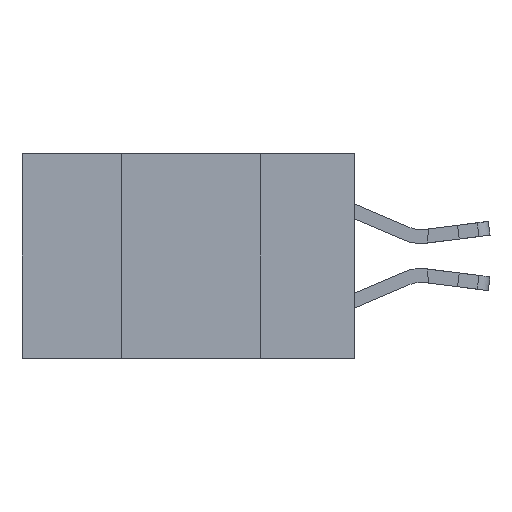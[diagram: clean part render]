
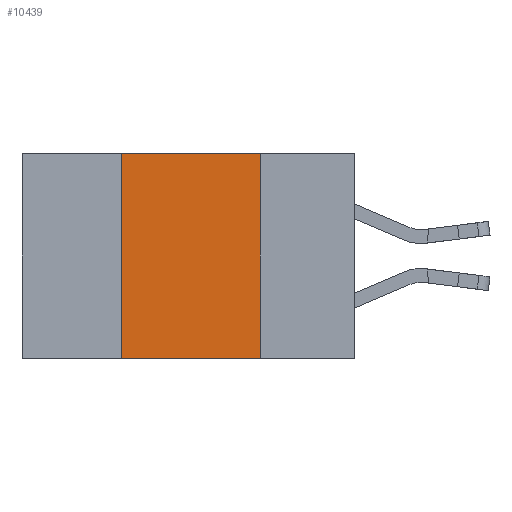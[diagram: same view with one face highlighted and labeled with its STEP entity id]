
A CAD part, left-side view. The second image highlights one B-rep face of the part: STEP entity #10439.
In plain terms, the highlighted planar face has unit normal (-1, 0, 0).
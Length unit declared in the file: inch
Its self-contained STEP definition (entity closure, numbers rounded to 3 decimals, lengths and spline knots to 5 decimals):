
#597 = CARTESIAN_POINT ( 'NONE',  ( 0., 0.42, -0.37 ) ) ;
#1867 = VERTEX_POINT ( 'NONE', #4042 ) ;
#1961 = CARTESIAN_POINT ( 'NONE',  ( 0., 0.6, 0. ) ) ;
#2543 = VERTEX_POINT ( 'NONE', #20258 ) ;
#2744 = EDGE_CURVE ( 'NONE', #1867, #18607, #13335, .T. ) ;
#3511 = EDGE_CURVE ( 'NONE', #3538, #18607, #19954, .T. ) ;
#3538 = VERTEX_POINT ( 'NONE', #597 ) ;
#4029 = DIRECTION ( 'NONE',  ( 0., 0., -1. ) ) ;
#4042 = CARTESIAN_POINT ( 'NONE',  ( 0., 0.17, 0. ) ) ;
#4999 = CARTESIAN_POINT ( 'NONE',  ( 0., 0.17, 0. ) ) ;
#5789 = CARTESIAN_POINT ( 'NONE',  ( 0., 0.17, -0.37 ) ) ;
#6169 = EDGE_LOOP ( 'NONE', ( #14895, #10889, #8827, #21037 ) ) ;
#6409 = DIRECTION ( 'NONE',  ( 1., 0., 0. ) ) ;
#6510 = EDGE_CURVE ( 'NONE', #2543, #1867, #17219, .T. ) ;
#6869 = VECTOR ( 'NONE', #18551, 39.37008 ) ;
#7229 = EDGE_CURVE ( 'NONE', #3538, #2543, #11378, .T. ) ;
#7869 = CARTESIAN_POINT ( 'NONE',  ( 0., 0.42, 0. ) ) ;
#8827 = ORIENTED_EDGE ( 'NONE', *, *, #7229, .F. ) ;
#10439 = ADVANCED_FACE ( 'NONE', ( #23257 ), #17344, .F. ) ;
#10889 = ORIENTED_EDGE ( 'NONE', *, *, #6510, .F. ) ;
#11378 = LINE ( 'NONE', #7869, #15757 ) ;
#12084 = DIRECTION ( 'NONE',  ( 0., -1., 0. ) ) ;
#13335 = LINE ( 'NONE', #4999, #17114 ) ;
#14699 = CARTESIAN_POINT ( 'NONE',  ( 0., 0.6, -0.37 ) ) ;
#14895 = ORIENTED_EDGE ( 'NONE', *, *, #2744, .F. ) ;
#15055 = VECTOR ( 'NONE', #12084, 39.37008 ) ;
#15757 = VECTOR ( 'NONE', #18860, 39.37008 ) ;
#17114 = VECTOR ( 'NONE', #4029, 39.37008 ) ;
#17219 = LINE ( 'NONE', #1961, #6869 ) ;
#17344 = PLANE ( 'NONE',  #21081 ) ;
#17433 = CARTESIAN_POINT ( 'NONE',  ( 0., 0.6, 0. ) ) ;
#18551 = DIRECTION ( 'NONE',  ( 0., -1., 0. ) ) ;
#18607 = VERTEX_POINT ( 'NONE', #5789 ) ;
#18860 = DIRECTION ( 'NONE',  ( 0., 0., 1. ) ) ;
#19287 = DIRECTION ( 'NONE',  ( 0., 0., -1. ) ) ;
#19954 = LINE ( 'NONE', #14699, #15055 ) ;
#20258 = CARTESIAN_POINT ( 'NONE',  ( 0., 0.42, 0. ) ) ;
#21037 = ORIENTED_EDGE ( 'NONE', *, *, #3511, .T. ) ;
#21081 = AXIS2_PLACEMENT_3D ( 'NONE', #17433, #6409, #19287 ) ;
#23257 = FACE_OUTER_BOUND ( 'NONE', #6169, .T. ) ;
